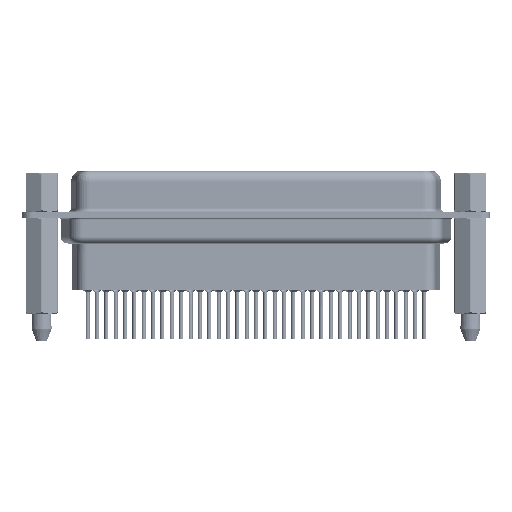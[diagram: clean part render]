
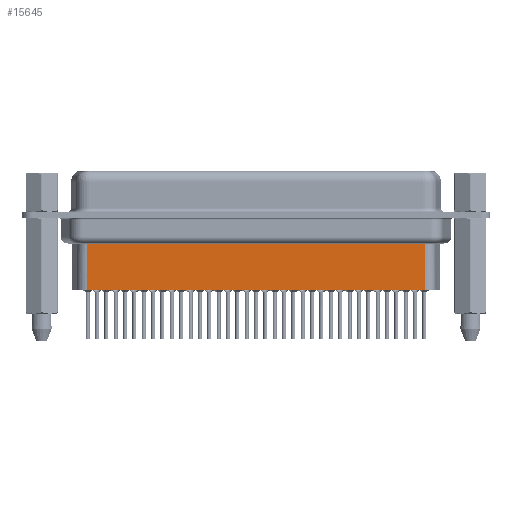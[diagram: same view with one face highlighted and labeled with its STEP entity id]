
A CAD part, front view. The second image highlights one B-rep face of the part: STEP entity #15645.
In plain terms, the highlighted planar face has unit normal (0, -1, 0).
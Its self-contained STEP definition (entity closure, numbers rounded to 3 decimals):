
#3313 = VERTEX_POINT ( 'NONE', #8404 ) ;
#4272 = EDGE_CURVE ( 'NONE', #17750, #30372, #36049, .T. ) ;
#5001 = DIRECTION ( 'NONE',  ( 0., 0., -1. ) ) ;
#5200 = EDGE_CURVE ( 'NONE', #28581, #17750, #26311, .T. ) ;
#8404 = CARTESIAN_POINT ( 'NONE',  ( 56.794, -3.5, -11.15 ) ) ;
#8571 = EDGE_LOOP ( 'NONE', ( #17776, #14758, #16110, #12912 ) ) ;
#9288 = CARTESIAN_POINT ( 'NONE',  ( 6.706, -3.5, -3.1 ) ) ;
#10488 = VECTOR ( 'NONE', #24920, 1000. ) ;
#10916 = DIRECTION ( 'NONE',  ( 1., 0., 0. ) ) ;
#11308 = DIRECTION ( 'NONE',  ( 0., -1., 0. ) ) ;
#12912 = ORIENTED_EDGE ( 'NONE', *, *, #31244, .F. ) ;
#12980 = LINE ( 'NONE', #13361, #10488 ) ;
#13361 = CARTESIAN_POINT ( 'NONE',  ( 6.706, -3.5, -11.15 ) ) ;
#14029 = PLANE ( 'NONE',  #34009 ) ;
#14758 = ORIENTED_EDGE ( 'NONE', *, *, #5200, .T. ) ;
#15645 = ADVANCED_FACE ( 'NONE', ( #38108 ), #14029, .T. ) ;
#16110 = ORIENTED_EDGE ( 'NONE', *, *, #4272, .T. ) ;
#16999 = VECTOR ( 'NONE', #28404, 1000. ) ;
#17249 = VECTOR ( 'NONE', #38236, 1000. ) ;
#17750 = VERTEX_POINT ( 'NONE', #28232 ) ;
#17776 = ORIENTED_EDGE ( 'NONE', *, *, #21634, .F. ) ;
#19621 = CARTESIAN_POINT ( 'NONE',  ( 6.706, -3.5, -11.15 ) ) ;
#21634 = EDGE_CURVE ( 'NONE', #28581, #3313, #25312, .T. ) ;
#23940 = CARTESIAN_POINT ( 'NONE',  ( 6.459, -3.5, -4.097 ) ) ;
#24298 = VECTOR ( 'NONE', #5001, 1000. ) ;
#24920 = DIRECTION ( 'NONE',  ( -1., 0., 0. ) ) ;
#25312 = LINE ( 'NONE', #25516, #24298 ) ;
#25516 = CARTESIAN_POINT ( 'NONE',  ( 56.794, -3.5, -3.1 ) ) ;
#25922 = CARTESIAN_POINT ( 'NONE',  ( 56.794, -3.5, -4.097 ) ) ;
#26311 = LINE ( 'NONE', #23940, #17249 ) ;
#28232 = CARTESIAN_POINT ( 'NONE',  ( 6.706, -3.5, -4.097 ) ) ;
#28404 = DIRECTION ( 'NONE',  ( 0., 0., -1. ) ) ;
#28581 = VERTEX_POINT ( 'NONE', #25922 ) ;
#30372 = VERTEX_POINT ( 'NONE', #19621 ) ;
#31244 = EDGE_CURVE ( 'NONE', #3313, #30372, #12980, .T. ) ;
#34009 = AXIS2_PLACEMENT_3D ( 'NONE', #37708, #11308, #10916 ) ;
#36049 = LINE ( 'NONE', #9288, #16999 ) ;
#37708 = CARTESIAN_POINT ( 'NONE',  ( 6.706, -3.5, -3.1 ) ) ;
#38108 = FACE_OUTER_BOUND ( 'NONE', #8571, .T. ) ;
#38236 = DIRECTION ( 'NONE',  ( -1., 0., 0. ) ) ;
